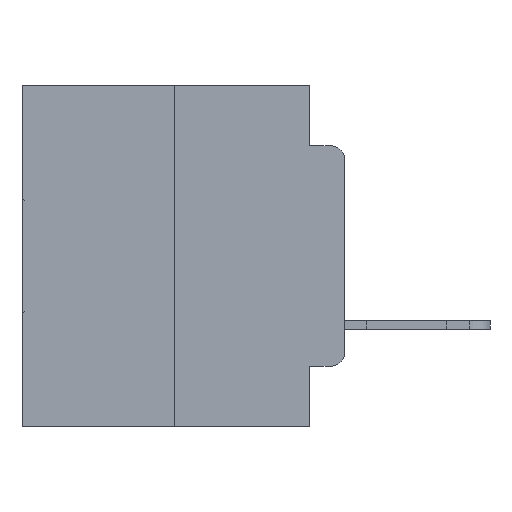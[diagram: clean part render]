
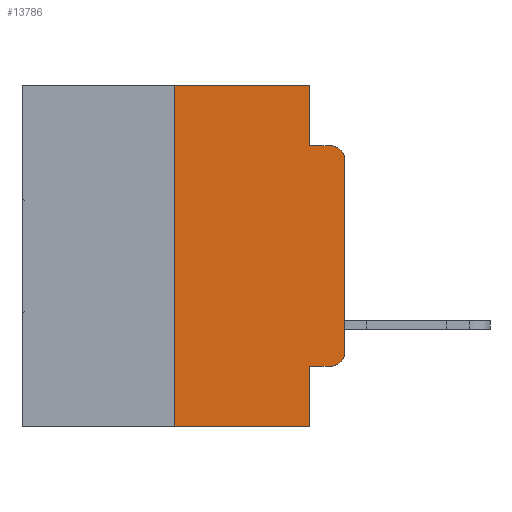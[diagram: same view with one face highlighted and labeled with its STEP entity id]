
A CAD part, left-side view. The second image highlights one B-rep face of the part: STEP entity #13786.
In plain terms, the highlighted planar face has unit normal (-1, 0, 0).
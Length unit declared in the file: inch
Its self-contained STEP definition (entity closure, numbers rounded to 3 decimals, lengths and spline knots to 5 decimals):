
#204 = DIRECTION ( 'NONE',  ( -1., 0., 0. ) ) ;
#295 = CARTESIAN_POINT ( 'NONE',  ( 0., 0.02, -0.3915 ) ) ;
#312 = VERTEX_POINT ( 'NONE', #538 ) ;
#397 = AXIS2_PLACEMENT_3D ( 'NONE', #14789, #19358, #14694 ) ;
#433 = LINE ( 'NONE', #11004, #24722 ) ;
#538 = CARTESIAN_POINT ( 'NONE',  ( 0., 0.051, 0. ) ) ;
#637 = CARTESIAN_POINT ( 'NONE',  ( 0., 0.25, 0. ) ) ;
#1083 = DIRECTION ( 'NONE',  ( 0., 0., -1. ) ) ;
#1312 = DIRECTION ( 'NONE',  ( 0., -1., 0. ) ) ;
#2510 = VERTEX_POINT ( 'NONE', #20170 ) ;
#2517 = LINE ( 'NONE', #19526, #21063 ) ;
#3031 = EDGE_CURVE ( 'NONE', #312, #25099, #7214, .T. ) ;
#3617 = VECTOR ( 'NONE', #26337, 39.37008 ) ;
#3646 = EDGE_CURVE ( 'NONE', #6938, #2510, #28499, .T. ) ;
#3680 = EDGE_CURVE ( 'NONE', #21206, #2510, #2517, .T. ) ;
#4304 = EDGE_CURVE ( 'NONE', #17011, #23001, #7857, .T. ) ;
#5200 = FACE_OUTER_BOUND ( 'NONE', #24221, .T. ) ;
#5439 = LINE ( 'NONE', #8670, #14009 ) ;
#5718 = CARTESIAN_POINT ( 'NONE',  ( 0., 0.473, 0. ) ) ;
#6229 = CARTESIAN_POINT ( 'NONE',  ( 0., 0.25, 0. ) ) ;
#6515 = DIRECTION ( 'NONE',  ( 0., -1., 0. ) ) ;
#6938 = VERTEX_POINT ( 'NONE', #9541 ) ;
#7214 = LINE ( 'NONE', #25136, #23593 ) ;
#7857 = CIRCLE ( 'NONE', #14992, 0.02 ) ;
#8223 = ORIENTED_EDGE ( 'NONE', *, *, #20572, .T. ) ;
#8670 = CARTESIAN_POINT ( 'NONE',  ( 0., 0.051, -0.0885 ) ) ;
#8684 = EDGE_CURVE ( 'NONE', #24533, #17011, #17645, .T. ) ;
#9541 = CARTESIAN_POINT ( 'NONE',  ( 0., 0.25, -0.5 ) ) ;
#9830 = CARTESIAN_POINT ( 'NONE',  ( 0., 0.02, -0.0885 ) ) ;
#10391 = CARTESIAN_POINT ( 'NONE',  ( 0., 0.473, -0.5 ) ) ;
#10695 = DIRECTION ( 'NONE',  ( 0., 0., -1. ) ) ;
#10715 = CIRCLE ( 'NONE', #13097, 0.02 ) ;
#11004 = CARTESIAN_POINT ( 'NONE',  ( 0., 0.051, -0.4115 ) ) ;
#13097 = AXIS2_PLACEMENT_3D ( 'NONE', #295, #204, #25045 ) ;
#13344 = DIRECTION ( 'NONE',  ( 0., 0., 1. ) ) ;
#13422 = CARTESIAN_POINT ( 'NONE',  ( 0., 0.02, -0.4115 ) ) ;
#13632 = VECTOR ( 'NONE', #14937, 39.37008 ) ;
#13786 = ADVANCED_FACE ( 'NONE', ( #5200 ), #21251, .F. ) ;
#14009 = VECTOR ( 'NONE', #24577, 39.37008 ) ;
#14097 = DIRECTION ( 'NONE',  ( 0., 0., -1. ) ) ;
#14208 = CARTESIAN_POINT ( 'NONE',  ( 0., 0.051, -0.4115 ) ) ;
#14556 = EDGE_CURVE ( 'NONE', #26090, #312, #19353, .T. ) ;
#14694 = DIRECTION ( 'NONE',  ( 0., 0., -1. ) ) ;
#14760 = CARTESIAN_POINT ( 'NONE',  ( 0., 0.02, -0.1085 ) ) ;
#14789 = CARTESIAN_POINT ( 'NONE',  ( 0., 0.473, 0. ) ) ;
#14937 = DIRECTION ( 'NONE',  ( 0., 0., 1. ) ) ;
#14992 = AXIS2_PLACEMENT_3D ( 'NONE', #14760, #24191, #1083 ) ;
#15303 = ORIENTED_EDGE ( 'NONE', *, *, #8684, .T. ) ;
#15387 = EDGE_CURVE ( 'NONE', #25099, #23001, #5439, .T. ) ;
#15759 = ORIENTED_EDGE ( 'NONE', *, *, #14556, .F. ) ;
#15801 = CARTESIAN_POINT ( 'NONE',  ( 0., 0., -0.3915 ) ) ;
#15997 = EDGE_CURVE ( 'NONE', #6938, #26090, #20007, .T. ) ;
#16009 = CARTESIAN_POINT ( 'NONE',  ( 0., 0., 0. ) ) ;
#17011 = VERTEX_POINT ( 'NONE', #25620 ) ;
#17645 = LINE ( 'NONE', #16009, #26131 ) ;
#19353 = LINE ( 'NONE', #5718, #23235 ) ;
#19358 = DIRECTION ( 'NONE',  ( 1., 0., 0. ) ) ;
#19526 = CARTESIAN_POINT ( 'NONE',  ( 0., 0.051, 0. ) ) ;
#19902 = ORIENTED_EDGE ( 'NONE', *, *, #3031, .F. ) ;
#20007 = LINE ( 'NONE', #637, #13632 ) ;
#20170 = CARTESIAN_POINT ( 'NONE',  ( 0., 0.051, -0.5 ) ) ;
#20572 = EDGE_CURVE ( 'NONE', #21206, #26712, #433, .T. ) ;
#21028 = ORIENTED_EDGE ( 'NONE', *, *, #3646, .T. ) ;
#21063 = VECTOR ( 'NONE', #10695, 39.37008 ) ;
#21206 = VERTEX_POINT ( 'NONE', #14208 ) ;
#21251 = PLANE ( 'NONE',  #397 ) ;
#22337 = ORIENTED_EDGE ( 'NONE', *, *, #15997, .F. ) ;
#23001 = VERTEX_POINT ( 'NONE', #9830 ) ;
#23235 = VECTOR ( 'NONE', #1312, 39.37008 ) ;
#23593 = VECTOR ( 'NONE', #14097, 39.37008 ) ;
#23594 = ORIENTED_EDGE ( 'NONE', *, *, #3680, .F. ) ;
#23907 = EDGE_CURVE ( 'NONE', #26712, #24533, #10715, .T. ) ;
#24191 = DIRECTION ( 'NONE',  ( -1., 0., 0. ) ) ;
#24221 = EDGE_LOOP ( 'NONE', ( #15303, #28035, #28286, #19902, #15759, #22337, #21028, #23594, #8223, #26835 ) ) ;
#24533 = VERTEX_POINT ( 'NONE', #15801 ) ;
#24577 = DIRECTION ( 'NONE',  ( 0., -1., 0. ) ) ;
#24722 = VECTOR ( 'NONE', #6515, 39.37008 ) ;
#25045 = DIRECTION ( 'NONE',  ( 0., 0., -1. ) ) ;
#25099 = VERTEX_POINT ( 'NONE', #27408 ) ;
#25136 = CARTESIAN_POINT ( 'NONE',  ( 0., 0.051, 0. ) ) ;
#25620 = CARTESIAN_POINT ( 'NONE',  ( 0., 0., -0.1085 ) ) ;
#26090 = VERTEX_POINT ( 'NONE', #6229 ) ;
#26131 = VECTOR ( 'NONE', #13344, 39.37008 ) ;
#26337 = DIRECTION ( 'NONE',  ( 0., -1., 0. ) ) ;
#26712 = VERTEX_POINT ( 'NONE', #13422 ) ;
#26835 = ORIENTED_EDGE ( 'NONE', *, *, #23907, .T. ) ;
#27408 = CARTESIAN_POINT ( 'NONE',  ( 0., 0.051, -0.0885 ) ) ;
#28035 = ORIENTED_EDGE ( 'NONE', *, *, #4304, .T. ) ;
#28286 = ORIENTED_EDGE ( 'NONE', *, *, #15387, .F. ) ;
#28499 = LINE ( 'NONE', #10391, #3617 ) ;
